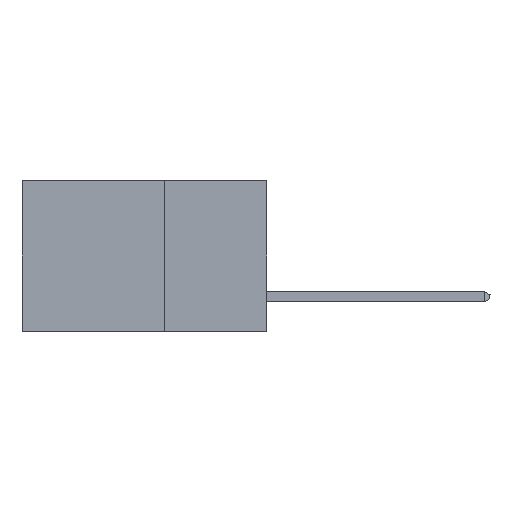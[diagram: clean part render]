
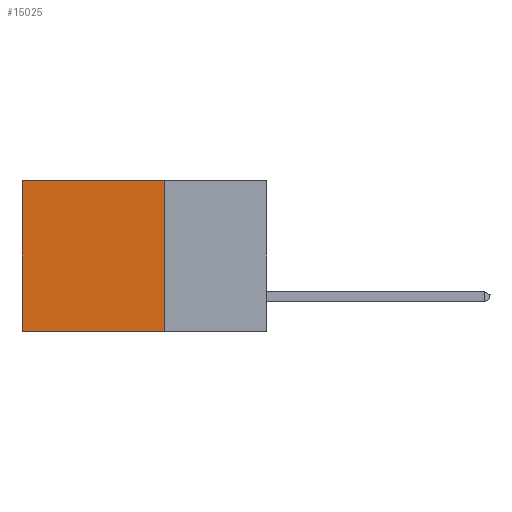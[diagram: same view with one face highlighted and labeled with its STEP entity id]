
A CAD part, left-side view. The second image highlights one B-rep face of the part: STEP entity #15025.
In plain terms, the highlighted planar face has unit normal (-1, 0, 0).
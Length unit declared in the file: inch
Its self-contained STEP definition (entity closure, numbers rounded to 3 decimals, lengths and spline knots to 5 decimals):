
#1932 = VECTOR ( 'NONE', #15924, 39.37008 ) ;
#3063 = EDGE_LOOP ( 'NONE', ( #44610, #3780, #8294, #46242 ) ) ;
#3460 = EDGE_CURVE ( 'NONE', #37362, #32492, #29458, .T. ) ;
#3567 = DIRECTION ( 'NONE',  ( 0., 1., 0. ) ) ;
#3780 = ORIENTED_EDGE ( 'NONE', *, *, #37854, .F. ) ;
#5726 = CARTESIAN_POINT ( 'NONE',  ( 0.2875, 0.25, 0. ) ) ;
#6569 = VERTEX_POINT ( 'NONE', #6650 ) ;
#6650 = CARTESIAN_POINT ( 'NONE',  ( 0.2875, 0.25, -0.37 ) ) ;
#8294 = ORIENTED_EDGE ( 'NONE', *, *, #23151, .F. ) ;
#8349 = DIRECTION ( 'NONE',  ( 0., 0., -1. ) ) ;
#8616 = CARTESIAN_POINT ( 'NONE',  ( 0.2875, 0.6, 0. ) ) ;
#8947 = DIRECTION ( 'NONE',  ( 0., 0., -1. ) ) ;
#9941 = VERTEX_POINT ( 'NONE', #27624 ) ;
#10389 = VECTOR ( 'NONE', #8349, 39.37008 ) ;
#12539 = CARTESIAN_POINT ( 'NONE',  ( 0.2875, 0.6, 0. ) ) ;
#15025 = ADVANCED_FACE ( 'NONE', ( #20532 ), #16351, .F. ) ;
#15924 = DIRECTION ( 'NONE',  ( 0., 1., 0. ) ) ;
#16351 = PLANE ( 'NONE',  #26587 ) ;
#20532 = FACE_OUTER_BOUND ( 'NONE', #3063, .T. ) ;
#23151 = EDGE_CURVE ( 'NONE', #37362, #6569, #28780, .T. ) ;
#23800 = CARTESIAN_POINT ( 'NONE',  ( 0.2875, 0.25, -0.37 ) ) ;
#24661 = EDGE_CURVE ( 'NONE', #32492, #9941, #45592, .T. ) ;
#24705 = DIRECTION ( 'NONE',  ( 1., 0., 0. ) ) ;
#25550 = DIRECTION ( 'NONE',  ( 0., 0., -1. ) ) ;
#26587 = AXIS2_PLACEMENT_3D ( 'NONE', #42976, #24705, #8947 ) ;
#27624 = CARTESIAN_POINT ( 'NONE',  ( 0.2875, 0.6, -0.37 ) ) ;
#28780 = LINE ( 'NONE', #43822, #39549 ) ;
#29458 = LINE ( 'NONE', #37344, #46816 ) ;
#32492 = VERTEX_POINT ( 'NONE', #8616 ) ;
#37344 = CARTESIAN_POINT ( 'NONE',  ( 0.2875, 0.25, 0. ) ) ;
#37362 = VERTEX_POINT ( 'NONE', #5726 ) ;
#37854 = EDGE_CURVE ( 'NONE', #6569, #9941, #38105, .T. ) ;
#38105 = LINE ( 'NONE', #23800, #1932 ) ;
#39549 = VECTOR ( 'NONE', #25550, 39.37008 ) ;
#42976 = CARTESIAN_POINT ( 'NONE',  ( 0.2875, 0.25, 0. ) ) ;
#43822 = CARTESIAN_POINT ( 'NONE',  ( 0.2875, 0.25, 0. ) ) ;
#44610 = ORIENTED_EDGE ( 'NONE', *, *, #24661, .T. ) ;
#45592 = LINE ( 'NONE', #12539, #10389 ) ;
#46242 = ORIENTED_EDGE ( 'NONE', *, *, #3460, .T. ) ;
#46816 = VECTOR ( 'NONE', #3567, 39.37008 ) ;
